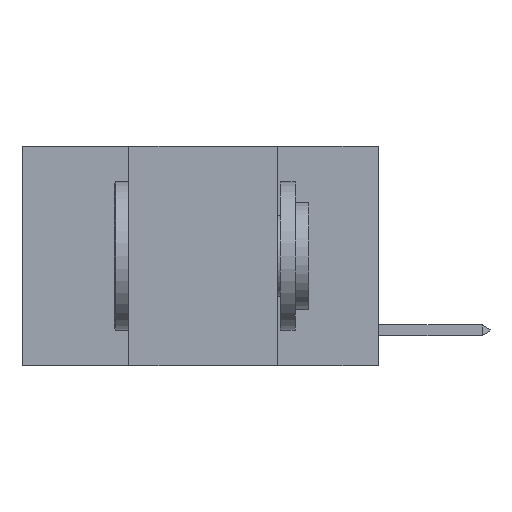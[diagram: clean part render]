
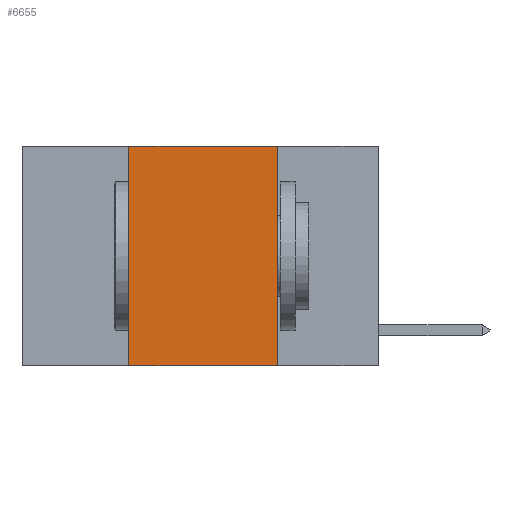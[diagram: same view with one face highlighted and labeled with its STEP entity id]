
A CAD part, left-side view. The second image highlights one B-rep face of the part: STEP entity #6655.
In plain terms, the highlighted planar face has unit normal (-1, 0, 0).
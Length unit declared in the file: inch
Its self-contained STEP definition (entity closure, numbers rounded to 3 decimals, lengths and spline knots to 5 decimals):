
#251 = PLANE ( 'NONE',  #13391 ) ;
#1195 = EDGE_CURVE ( 'NONE', #4616, #13283, #14208, .T. ) ;
#2480 = EDGE_CURVE ( 'NONE', #9998, #10262, #19060, .T. ) ;
#2511 = VECTOR ( 'NONE', #5608, 39.37008 ) ;
#3299 = CARTESIAN_POINT ( 'NONE',  ( 0., 0.42, 0. ) ) ;
#3340 = DIRECTION ( 'NONE',  ( 1., 0., 0. ) ) ;
#4616 = VERTEX_POINT ( 'NONE', #10604 ) ;
#4644 = VECTOR ( 'NONE', #4875, 39.37008 ) ;
#4875 = DIRECTION ( 'NONE',  ( 0., 0., 1. ) ) ;
#5608 = DIRECTION ( 'NONE',  ( 0., -1., 0. ) ) ;
#6655 = ADVANCED_FACE ( 'NONE', ( #14391 ), #251, .F. ) ;
#7037 = VECTOR ( 'NONE', #7885, 39.37008 ) ;
#7885 = DIRECTION ( 'NONE',  ( 0., -1., 0. ) ) ;
#8000 = CARTESIAN_POINT ( 'NONE',  ( 0., 0.6, -0.37 ) ) ;
#9939 = CARTESIAN_POINT ( 'NONE',  ( 0., 0.17, -0.37 ) ) ;
#9998 = VERTEX_POINT ( 'NONE', #10759 ) ;
#10262 = VERTEX_POINT ( 'NONE', #9939 ) ;
#10604 = CARTESIAN_POINT ( 'NONE',  ( 0., 0.42, 0. ) ) ;
#10759 = CARTESIAN_POINT ( 'NONE',  ( 0., 0.42, -0.37 ) ) ;
#10913 = VECTOR ( 'NONE', #11920, 39.37008 ) ;
#11655 = ORIENTED_EDGE ( 'NONE', *, *, #12755, .F. ) ;
#11859 = CARTESIAN_POINT ( 'NONE',  ( 0., 0.17, 0. ) ) ;
#11920 = DIRECTION ( 'NONE',  ( 0., 0., -1. ) ) ;
#12485 = CARTESIAN_POINT ( 'NONE',  ( 0., 0.6, 0. ) ) ;
#12738 = LINE ( 'NONE', #3299, #4644 ) ;
#12755 = EDGE_CURVE ( 'NONE', #13283, #10262, #14972, .T. ) ;
#13098 = ORIENTED_EDGE ( 'NONE', *, *, #2480, .T. ) ;
#13283 = VERTEX_POINT ( 'NONE', #16125 ) ;
#13391 = AXIS2_PLACEMENT_3D ( 'NONE', #12485, #3340, #14030 ) ;
#14030 = DIRECTION ( 'NONE',  ( 0., 0., -1. ) ) ;
#14208 = LINE ( 'NONE', #14636, #2511 ) ;
#14391 = FACE_OUTER_BOUND ( 'NONE', #15961, .T. ) ;
#14636 = CARTESIAN_POINT ( 'NONE',  ( 0., 0.6, 0. ) ) ;
#14972 = LINE ( 'NONE', #11859, #10913 ) ;
#15511 = EDGE_CURVE ( 'NONE', #9998, #4616, #12738, .T. ) ;
#15682 = ORIENTED_EDGE ( 'NONE', *, *, #1195, .F. ) ;
#15961 = EDGE_LOOP ( 'NONE', ( #11655, #15682, #16150, #13098 ) ) ;
#16125 = CARTESIAN_POINT ( 'NONE',  ( 0., 0.17, 0. ) ) ;
#16150 = ORIENTED_EDGE ( 'NONE', *, *, #15511, .F. ) ;
#19060 = LINE ( 'NONE', #8000, #7037 ) ;
